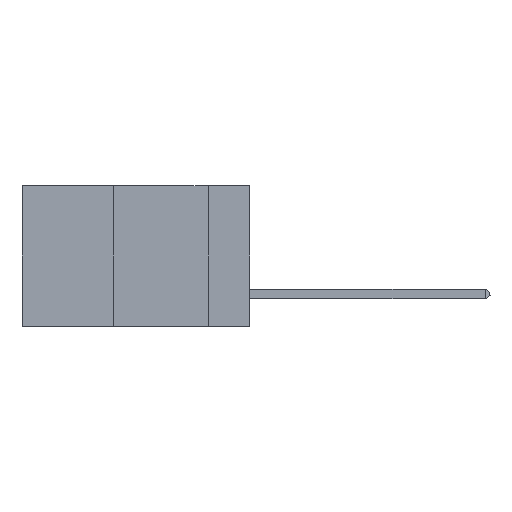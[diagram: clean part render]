
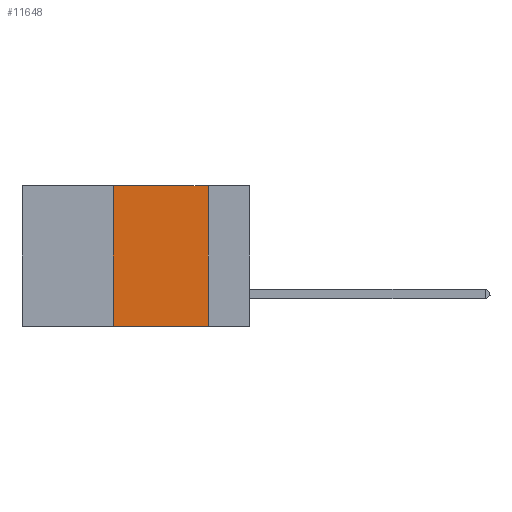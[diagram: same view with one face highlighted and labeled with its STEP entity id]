
A CAD part, left-side view. The second image highlights one B-rep face of the part: STEP entity #11648.
In plain terms, the highlighted planar face has unit normal (-1, 0, 0).
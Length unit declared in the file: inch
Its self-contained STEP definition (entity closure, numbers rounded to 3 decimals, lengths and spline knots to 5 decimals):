
#1155 = DIRECTION ( 'NONE',  ( 1., 0., 0. ) ) ;
#1244 = CARTESIAN_POINT ( 'NONE',  ( 0., 0.6, 0. ) ) ;
#1727 = VERTEX_POINT ( 'NONE', #31482 ) ;
#2576 = EDGE_CURVE ( 'NONE', #19362, #5689, #29293, .T. ) ;
#3486 = EDGE_CURVE ( 'NONE', #5689, #30934, #29793, .T. ) ;
#4791 = DIRECTION ( 'NONE',  ( 0., 0., -1. ) ) ;
#5689 = VERTEX_POINT ( 'NONE', #37318 ) ;
#7985 = CARTESIAN_POINT ( 'NONE',  ( 0., 0.36, 0. ) ) ;
#8799 = DIRECTION ( 'NONE',  ( 0., -1., 0. ) ) ;
#11648 = ADVANCED_FACE ( 'NONE', ( #40458 ), #43746, .F. ) ;
#11714 = CARTESIAN_POINT ( 'NONE',  ( 0., 0.6, 0. ) ) ;
#13780 = LINE ( 'NONE', #19906, #23969 ) ;
#19362 = VERTEX_POINT ( 'NONE', #23614 ) ;
#19906 = CARTESIAN_POINT ( 'NONE',  ( 0., 0.11, 0. ) ) ;
#20366 = EDGE_CURVE ( 'NONE', #19362, #1727, #34379, .T. ) ;
#20724 = DIRECTION ( 'NONE',  ( 0., -1., 0. ) ) ;
#23614 = CARTESIAN_POINT ( 'NONE',  ( 0., 0.36, -0.37 ) ) ;
#23969 = VECTOR ( 'NONE', #30543, 39.37008 ) ;
#25206 = ORIENTED_EDGE ( 'NONE', *, *, #2576, .F. ) ;
#29293 = LINE ( 'NONE', #7985, #39903 ) ;
#29318 = DIRECTION ( 'NONE',  ( 0., 0., 1. ) ) ;
#29793 = LINE ( 'NONE', #1244, #38149 ) ;
#30543 = DIRECTION ( 'NONE',  ( 0., 0., -1. ) ) ;
#30934 = VERTEX_POINT ( 'NONE', #32975 ) ;
#31482 = CARTESIAN_POINT ( 'NONE',  ( 0., 0.11, -0.37 ) ) ;
#32831 = EDGE_CURVE ( 'NONE', #30934, #1727, #13780, .T. ) ;
#32975 = CARTESIAN_POINT ( 'NONE',  ( 0., 0.11, 0. ) ) ;
#34379 = LINE ( 'NONE', #45526, #40491 ) ;
#37226 = ORIENTED_EDGE ( 'NONE', *, *, #3486, .F. ) ;
#37318 = CARTESIAN_POINT ( 'NONE',  ( 0., 0.36, 0. ) ) ;
#37956 = EDGE_LOOP ( 'NONE', ( #38000, #37226, #25206, #45417 ) ) ;
#38000 = ORIENTED_EDGE ( 'NONE', *, *, #32831, .F. ) ;
#38149 = VECTOR ( 'NONE', #8799, 39.37008 ) ;
#39903 = VECTOR ( 'NONE', #29318, 39.37008 ) ;
#40046 = AXIS2_PLACEMENT_3D ( 'NONE', #11714, #1155, #4791 ) ;
#40458 = FACE_OUTER_BOUND ( 'NONE', #37956, .T. ) ;
#40491 = VECTOR ( 'NONE', #20724, 39.37008 ) ;
#43746 = PLANE ( 'NONE',  #40046 ) ;
#45417 = ORIENTED_EDGE ( 'NONE', *, *, #20366, .T. ) ;
#45526 = CARTESIAN_POINT ( 'NONE',  ( 0., 0.6, -0.37 ) ) ;
